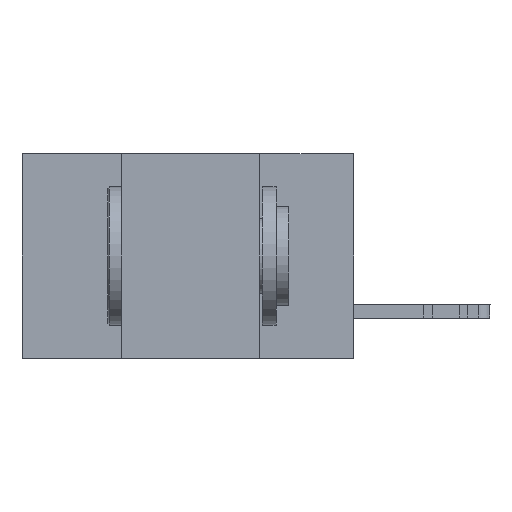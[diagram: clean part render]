
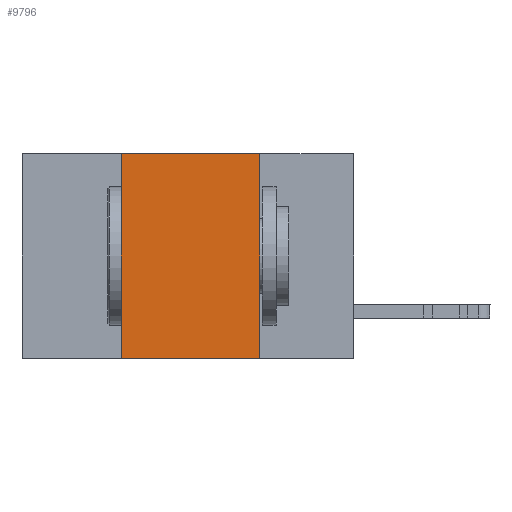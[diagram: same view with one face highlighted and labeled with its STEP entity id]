
A CAD part, left-side view. The second image highlights one B-rep face of the part: STEP entity #9796.
In plain terms, the highlighted planar face has unit normal (-1, 0, 0).
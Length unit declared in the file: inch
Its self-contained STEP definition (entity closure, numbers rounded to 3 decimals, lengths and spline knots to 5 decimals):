
#112 = LINE ( 'NONE', #14484, #8169 ) ;
#1241 = CARTESIAN_POINT ( 'NONE',  ( 0., 0.17, 0. ) ) ;
#1414 = VERTEX_POINT ( 'NONE', #5184 ) ;
#2529 = ORIENTED_EDGE ( 'NONE', *, *, #35143, .F. ) ;
#2544 = LINE ( 'NONE', #10068, #12297 ) ;
#2681 = PLANE ( 'NONE',  #35034 ) ;
#5184 = CARTESIAN_POINT ( 'NONE',  ( 0., 0.42, -0.37 ) ) ;
#5335 = VERTEX_POINT ( 'NONE', #24609 ) ;
#6460 = CARTESIAN_POINT ( 'NONE',  ( 0., 0.6, 0. ) ) ;
#6970 = CARTESIAN_POINT ( 'NONE',  ( 0., 0.42, 0. ) ) ;
#8159 = VERTEX_POINT ( 'NONE', #44434 ) ;
#8169 = VECTOR ( 'NONE', #21993, 39.37008 ) ;
#9796 = ADVANCED_FACE ( 'NONE', ( #31845 ), #2681, .F. ) ;
#10068 = CARTESIAN_POINT ( 'NONE',  ( 0., 0.6, 0. ) ) ;
#11099 = DIRECTION ( 'NONE',  ( 0., -1., 0. ) ) ;
#12297 = VECTOR ( 'NONE', #13144, 39.37008 ) ;
#13144 = DIRECTION ( 'NONE',  ( 0., -1., 0. ) ) ;
#14484 = CARTESIAN_POINT ( 'NONE',  ( 0., 0.17, 0. ) ) ;
#16826 = CARTESIAN_POINT ( 'NONE',  ( 0., 0.6, -0.37 ) ) ;
#20504 = VECTOR ( 'NONE', #11099, 39.37008 ) ;
#20552 = DIRECTION ( 'NONE',  ( 0., 0., -1. ) ) ;
#21993 = DIRECTION ( 'NONE',  ( 0., 0., -1. ) ) ;
#24609 = CARTESIAN_POINT ( 'NONE',  ( 0., 0.42, 0. ) ) ;
#25026 = VERTEX_POINT ( 'NONE', #1241 ) ;
#29486 = ORIENTED_EDGE ( 'NONE', *, *, #37048, .F. ) ;
#29981 = EDGE_CURVE ( 'NONE', #1414, #5335, #45636, .T. ) ;
#31845 = FACE_OUTER_BOUND ( 'NONE', #41152, .T. ) ;
#35034 = AXIS2_PLACEMENT_3D ( 'NONE', #6460, #39155, #20552 ) ;
#35143 = EDGE_CURVE ( 'NONE', #5335, #25026, #2544, .T. ) ;
#36875 = VECTOR ( 'NONE', #39444, 39.37008 ) ;
#37048 = EDGE_CURVE ( 'NONE', #25026, #8159, #112, .T. ) ;
#38479 = LINE ( 'NONE', #16826, #20504 ) ;
#39155 = DIRECTION ( 'NONE',  ( 1., 0., 0. ) ) ;
#39444 = DIRECTION ( 'NONE',  ( 0., 0., 1. ) ) ;
#40892 = ORIENTED_EDGE ( 'NONE', *, *, #41826, .T. ) ;
#41152 = EDGE_LOOP ( 'NONE', ( #29486, #2529, #45004, #40892 ) ) ;
#41826 = EDGE_CURVE ( 'NONE', #1414, #8159, #38479, .T. ) ;
#44434 = CARTESIAN_POINT ( 'NONE',  ( 0., 0.17, -0.37 ) ) ;
#45004 = ORIENTED_EDGE ( 'NONE', *, *, #29981, .F. ) ;
#45636 = LINE ( 'NONE', #6970, #36875 ) ;
